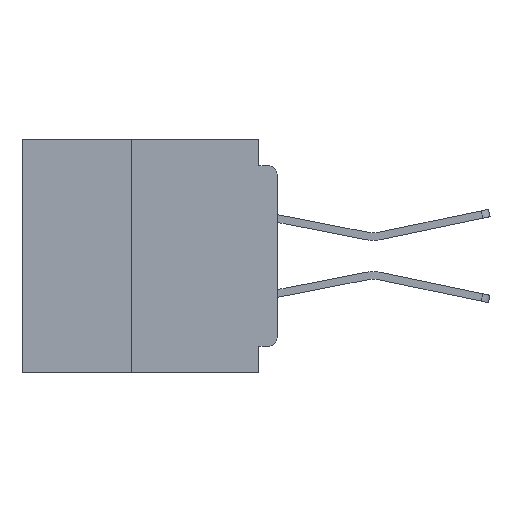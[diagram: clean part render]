
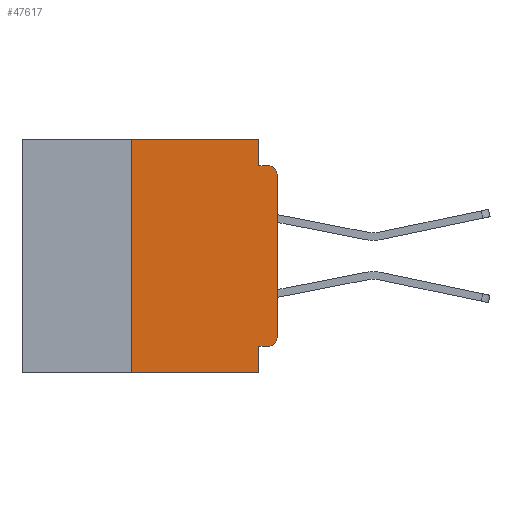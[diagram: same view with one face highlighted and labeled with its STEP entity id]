
A CAD part, left-side view. The second image highlights one B-rep face of the part: STEP entity #47617.
In plain terms, the highlighted planar face has unit normal (-1, 0, 0).
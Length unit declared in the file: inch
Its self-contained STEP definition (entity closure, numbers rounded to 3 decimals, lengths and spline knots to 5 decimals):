
#806 = LINE ( 'NONE', #23492, #49695 ) ;
#870 = DIRECTION ( 'NONE',  ( 1., 0., 0. ) ) ;
#1053 = VECTOR ( 'NONE', #39361, 39.37008 ) ;
#1060 = LINE ( 'NONE', #3120, #20437 ) ;
#2238 = CARTESIAN_POINT ( 'NONE',  ( 0., 0.031, -0.4 ) ) ;
#2241 = DIRECTION ( 'NONE',  ( 0., 1., 0. ) ) ;
#3042 = EDGE_CURVE ( 'NONE', #38785, #26231, #25858, .T. ) ;
#3081 = EDGE_LOOP ( 'NONE', ( #28672, #37128, #36278, #15337, #16315, #36676, #46198, #30651, #38530, #15783 ) ) ;
#3120 = CARTESIAN_POINT ( 'NONE',  ( 0., 0.437, -0.4 ) ) ;
#3851 = EDGE_CURVE ( 'NONE', #38785, #45816, #19792, .T. ) ;
#5461 = CIRCLE ( 'NONE', #29401, 0.015 ) ;
#6553 = EDGE_CURVE ( 'NONE', #26231, #27935, #24958, .T. ) ;
#7807 = LINE ( 'NONE', #39225, #46459 ) ;
#8082 = DIRECTION ( 'NONE',  ( 0., -1., 0. ) ) ;
#9024 = EDGE_CURVE ( 'NONE', #10527, #49753, #31967, .T. ) ;
#9395 = VECTOR ( 'NONE', #25317, 39.37008 ) ;
#10527 = VERTEX_POINT ( 'NONE', #33506 ) ;
#10854 = VERTEX_POINT ( 'NONE', #35343 ) ;
#10947 = DIRECTION ( 'NONE',  ( -1., 0., 0. ) ) ;
#12217 = CARTESIAN_POINT ( 'NONE',  ( 0., 0.031, -0.045 ) ) ;
#14639 = VECTOR ( 'NONE', #17161, 39.37008 ) ;
#15337 = ORIENTED_EDGE ( 'NONE', *, *, #32343, .F. ) ;
#15783 = ORIENTED_EDGE ( 'NONE', *, *, #3851, .T. ) ;
#15929 = CARTESIAN_POINT ( 'NONE',  ( 0., 0., -0.34 ) ) ;
#16315 = ORIENTED_EDGE ( 'NONE', *, *, #49492, .F. ) ;
#17161 = DIRECTION ( 'NONE',  ( 0., 0., -1. ) ) ;
#18124 = VECTOR ( 'NONE', #8082, 39.37008 ) ;
#18277 = DIRECTION ( 'NONE',  ( -1., 0., 0. ) ) ;
#18665 = AXIS2_PLACEMENT_3D ( 'NONE', #47120, #870, #27957 ) ;
#19712 = LINE ( 'NONE', #48347, #9395 ) ;
#19769 = CARTESIAN_POINT ( 'NONE',  ( 0., 0.25, -0.4 ) ) ;
#19792 = CIRCLE ( 'NONE', #46647, 0.015 ) ;
#19978 = DIRECTION ( 'NONE',  ( 0., -1., 0. ) ) ;
#20437 = VECTOR ( 'NONE', #49504, 39.37008 ) ;
#20438 = CARTESIAN_POINT ( 'NONE',  ( 0., 0.031, 0. ) ) ;
#21894 = CARTESIAN_POINT ( 'NONE',  ( 0., 0.031, -0.355 ) ) ;
#22074 = EDGE_CURVE ( 'NONE', #24666, #28735, #28417, .T. ) ;
#23492 = CARTESIAN_POINT ( 'NONE',  ( 0., 0., 0. ) ) ;
#24643 = VECTOR ( 'NONE', #2241, 39.37008 ) ;
#24666 = VERTEX_POINT ( 'NONE', #12217 ) ;
#24958 = LINE ( 'NONE', #44292, #14639 ) ;
#25317 = DIRECTION ( 'NONE',  ( 0., 0., -1. ) ) ;
#25858 = LINE ( 'NONE', #36889, #24643 ) ;
#26231 = VERTEX_POINT ( 'NONE', #21894 ) ;
#27935 = VERTEX_POINT ( 'NONE', #2238 ) ;
#27957 = DIRECTION ( 'NONE',  ( 0., 0., -1. ) ) ;
#28417 = LINE ( 'NONE', #31304, #18124 ) ;
#28672 = ORIENTED_EDGE ( 'NONE', *, *, #38041, .T. ) ;
#28735 = VERTEX_POINT ( 'NONE', #42704 ) ;
#29401 = AXIS2_PLACEMENT_3D ( 'NONE', #41399, #18277, #45224 ) ;
#30363 = FACE_OUTER_BOUND ( 'NONE', #3081, .T. ) ;
#30651 = ORIENTED_EDGE ( 'NONE', *, *, #6553, .F. ) ;
#31212 = EDGE_CURVE ( 'NONE', #10527, #27935, #1060, .T. ) ;
#31304 = CARTESIAN_POINT ( 'NONE',  ( 0., 0., -0.045 ) ) ;
#31967 = LINE ( 'NONE', #19769, #1053 ) ;
#32343 = EDGE_CURVE ( 'NONE', #40011, #24666, #19712, .T. ) ;
#33506 = CARTESIAN_POINT ( 'NONE',  ( 0., 0.25, -0.4 ) ) ;
#34136 = CARTESIAN_POINT ( 'NONE',  ( 0., 0.015, -0.34 ) ) ;
#35343 = CARTESIAN_POINT ( 'NONE',  ( 0., 0., -0.06 ) ) ;
#36278 = ORIENTED_EDGE ( 'NONE', *, *, #22074, .F. ) ;
#36676 = ORIENTED_EDGE ( 'NONE', *, *, #9024, .F. ) ;
#36889 = CARTESIAN_POINT ( 'NONE',  ( 0., 0., -0.355 ) ) ;
#37128 = ORIENTED_EDGE ( 'NONE', *, *, #39634, .T. ) ;
#37990 = DIRECTION ( 'NONE',  ( 0., 0., -1. ) ) ;
#38041 = EDGE_CURVE ( 'NONE', #45816, #10854, #806, .T. ) ;
#38530 = ORIENTED_EDGE ( 'NONE', *, *, #3042, .F. ) ;
#38785 = VERTEX_POINT ( 'NONE', #43969 ) ;
#39001 = DIRECTION ( 'NONE',  ( 0., 0., 1. ) ) ;
#39225 = CARTESIAN_POINT ( 'NONE',  ( 0., 0.437, 0. ) ) ;
#39361 = DIRECTION ( 'NONE',  ( 0., 0., 1. ) ) ;
#39634 = EDGE_CURVE ( 'NONE', #10854, #28735, #5461, .T. ) ;
#40011 = VERTEX_POINT ( 'NONE', #20438 ) ;
#40892 = CARTESIAN_POINT ( 'NONE',  ( 0., 0.25, 0. ) ) ;
#41399 = CARTESIAN_POINT ( 'NONE',  ( 0., 0.015, -0.06 ) ) ;
#42704 = CARTESIAN_POINT ( 'NONE',  ( 0., 0.015, -0.045 ) ) ;
#43261 = PLANE ( 'NONE',  #18665 ) ;
#43969 = CARTESIAN_POINT ( 'NONE',  ( 0., 0.015, -0.355 ) ) ;
#44292 = CARTESIAN_POINT ( 'NONE',  ( 0., 0.031, -0.4 ) ) ;
#45224 = DIRECTION ( 'NONE',  ( 0., 0., -1. ) ) ;
#45816 = VERTEX_POINT ( 'NONE', #15929 ) ;
#46198 = ORIENTED_EDGE ( 'NONE', *, *, #31212, .T. ) ;
#46459 = VECTOR ( 'NONE', #19978, 39.37008 ) ;
#46647 = AXIS2_PLACEMENT_3D ( 'NONE', #34136, #10947, #37990 ) ;
#47120 = CARTESIAN_POINT ( 'NONE',  ( 0., 0.437, 0. ) ) ;
#47617 = ADVANCED_FACE ( 'NONE', ( #30363 ), #43261, .F. ) ;
#48347 = CARTESIAN_POINT ( 'NONE',  ( 0., 0.031, 0. ) ) ;
#49492 = EDGE_CURVE ( 'NONE', #49753, #40011, #7807, .T. ) ;
#49504 = DIRECTION ( 'NONE',  ( 0., -1., 0. ) ) ;
#49695 = VECTOR ( 'NONE', #39001, 39.37008 ) ;
#49753 = VERTEX_POINT ( 'NONE', #40892 ) ;
